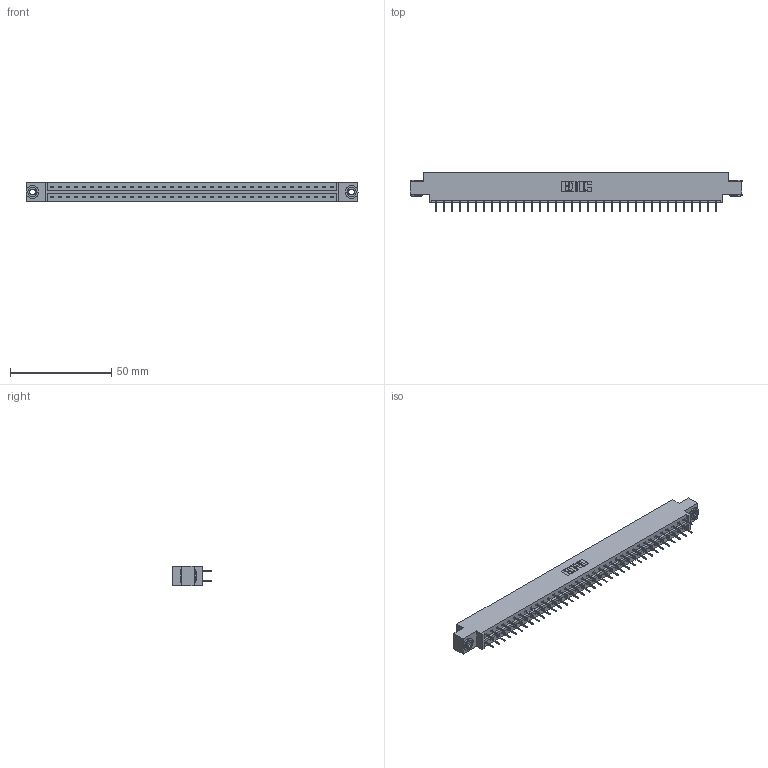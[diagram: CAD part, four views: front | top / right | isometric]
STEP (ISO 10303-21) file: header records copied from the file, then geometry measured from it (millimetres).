
FILE_DESCRIPTION (( 'STEP AP203' ), '1' );
FILE_NAME ('333-072-524-803.STEP', '2018-08-04T20:42:14', ( '' ), ( '' ), 'SwSTEP 2.0', 'SolidWorks 2016', '' );
FILE_SCHEMA (( 'CONFIG_CONTROL_DESIGN' ));
Length unit declared in the file: inch
Products named in the file (4): 345-250-002_345-250-002-102; 333-072-524-803; 333 Part_Offset - .156 Dia - TH; 345-292-001_345-293-124
Assembly tree (75 placements, depth 2):
  333-072-524-803
    333 Part_Offset - .156 Dia - TH
    345-292-001_345-293-124  x72
    345-250-002_345-250-002-102  x2
Bounding box: 164.19 x 19.69 x 9.4 mm (x, y, z)
Volume: 16388.9 mm3; surface area: 19426 mm2
Topology: 75 solids, 75 shells, 4188 faces, 11847 edges, 7606 vertices
Faces by surface type: plane 3108, cylinder 1072, cone 8
Entity records: 24792 total; most frequent: CARTESIAN_POINT 4093, ORIENTED_EDGE 4022, DIRECTION 3541, EDGE_CURVE 2011, LINE 1863, VECTOR 1863, VERTEX_POINT 1334, AXIS2_PLACEMENT_3D 839
